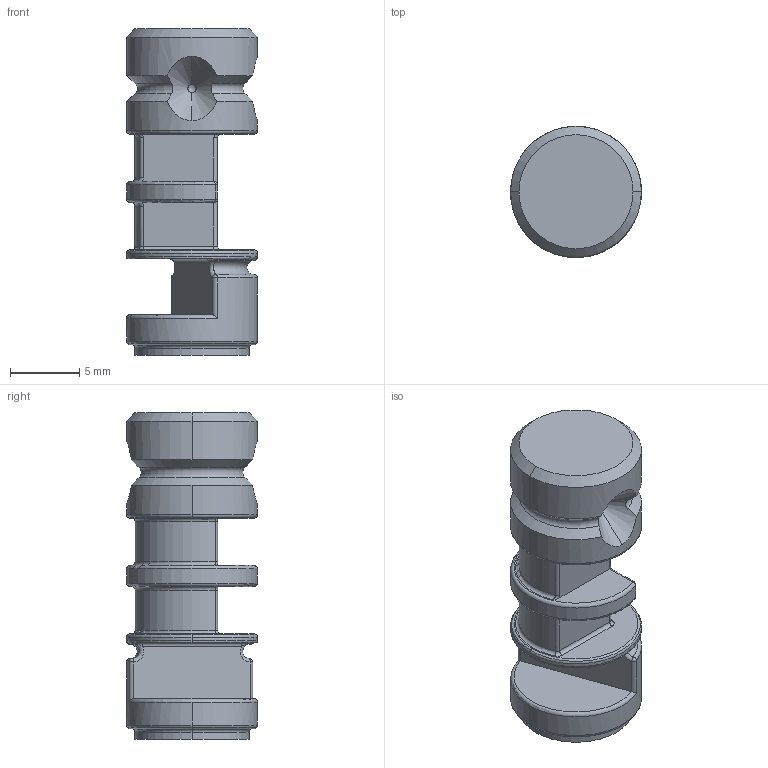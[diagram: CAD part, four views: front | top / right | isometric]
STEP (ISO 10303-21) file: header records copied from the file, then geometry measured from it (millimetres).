
FILE_DESCRIPTION((''),'2;1');
FILE_NAME('SOLID1','2019-01-20T17:52:54',('Cust'),(''),'CREO PARAMETRIC BY PTC INC, 2018300','CREO PARAMETRIC BY PTC INC, 2018300','');
FILE_SCHEMA(('AUTOMOTIVE_DESIGN { 1 0 10303 214 1 1 1 1 }'));
Length unit declared in the file: inch
Products named in the file (1): SOLID1
Bounding box: 9.47 x 9.47 x 23.62 mm (x, y, z)
Volume: 1142.7 mm3; surface area: 941.9 mm2
Topology: 1 solids, 1 shells, 113 faces, 319 edges, 211 vertices
Faces by surface type: torus 37, cylinder 31, cone 14, plane 13, sphere 9, bspline 9
Entity records: 5395 total; most frequent: CARTESIAN_POINT 1444, ORIENTED_EDGE 638, DIRECTION 626, PRESENTATION_STYLE_ASSIGNMENT 320, STYLED_ITEM 320, CURVE_STYLE 319, EDGE_CURVE 319, AXIS2_PLACEMENT_3D 284
